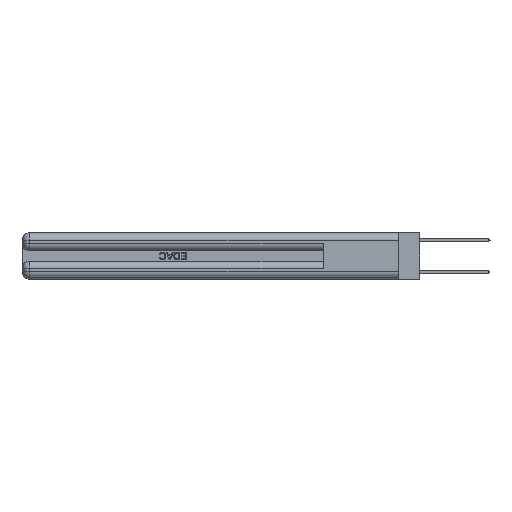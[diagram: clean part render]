
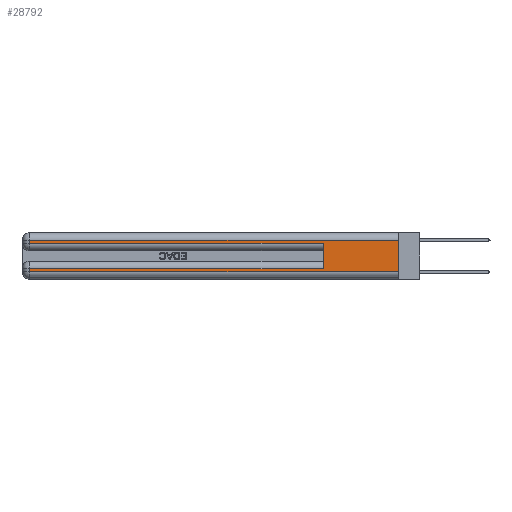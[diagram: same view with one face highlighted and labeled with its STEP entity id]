
A CAD part, left-side view. The second image highlights one B-rep face of the part: STEP entity #28792.
In plain terms, the highlighted planar face has unit normal (-1, 0, 0).
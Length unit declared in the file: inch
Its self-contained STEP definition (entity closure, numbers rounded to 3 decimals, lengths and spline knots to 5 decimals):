
#132 = LINE ( 'NONE', #19905, #26265 ) ;
#1682 = VERTEX_POINT ( 'NONE', #32365 ) ;
#1785 = ORIENTED_EDGE ( 'NONE', *, *, #12362, .T. ) ;
#2155 = EDGE_CURVE ( 'NONE', #25075, #1682, #28008, .T. ) ;
#2584 = LINE ( 'NONE', #23247, #15308 ) ;
#3776 = ORIENTED_EDGE ( 'NONE', *, *, #16377, .T. ) ;
#3825 = EDGE_CURVE ( 'NONE', #22819, #23001, #2584, .T. ) ;
#4511 = VERTEX_POINT ( 'NONE', #26385 ) ;
#4681 = DIRECTION ( 'NONE',  ( 0., 1., 0. ) ) ;
#5069 = EDGE_LOOP ( 'NONE', ( #28357, #23232, #3776, #12104, #25578, #13677, #1785, #31104 ) ) ;
#6188 = VERTEX_POINT ( 'NONE', #31157 ) ;
#6402 = CARTESIAN_POINT ( 'NONE',  ( 0., 0.6, 0.085 ) ) ;
#7669 = CARTESIAN_POINT ( 'NONE',  ( 0., 2.94, 0.06 ) ) ;
#7824 = VECTOR ( 'NONE', #28926, 39.37008 ) ;
#8677 = DIRECTION ( 'NONE',  ( 1., 0., 0. ) ) ;
#9078 = CARTESIAN_POINT ( 'NONE',  ( 0., 0., 0.06 ) ) ;
#10394 = LINE ( 'NONE', #29727, #29802 ) ;
#10498 = DIRECTION ( 'NONE',  ( 0., 0., 1. ) ) ;
#10641 = EDGE_CURVE ( 'NONE', #22819, #6188, #132, .T. ) ;
#10685 = LINE ( 'NONE', #29295, #30100 ) ;
#12054 = CARTESIAN_POINT ( 'NONE',  ( 0., 0.6, 0.285 ) ) ;
#12104 = ORIENTED_EDGE ( 'NONE', *, *, #23173, .T. ) ;
#12362 = EDGE_CURVE ( 'NONE', #6188, #28641, #14928, .T. ) ;
#13038 = AXIS2_PLACEMENT_3D ( 'NONE', #18746, #8677, #26354 ) ;
#13677 = ORIENTED_EDGE ( 'NONE', *, *, #10641, .T. ) ;
#14040 = EDGE_CURVE ( 'NONE', #28641, #18282, #28649, .T. ) ;
#14707 = EDGE_CURVE ( 'NONE', #25075, #18282, #10394, .T. ) ;
#14928 = LINE ( 'NONE', #30890, #26773 ) ;
#15273 = CARTESIAN_POINT ( 'NONE',  ( 0., 0., 0.285 ) ) ;
#15308 = VECTOR ( 'NONE', #10498, 39.37008 ) ;
#16315 = CARTESIAN_POINT ( 'NONE',  ( 0., 0., 0.31 ) ) ;
#16377 = EDGE_CURVE ( 'NONE', #1682, #4511, #10685, .T. ) ;
#17431 = CARTESIAN_POINT ( 'NONE',  ( 0., 0., 0.06 ) ) ;
#18282 = VERTEX_POINT ( 'NONE', #9078 ) ;
#18443 = LINE ( 'NONE', #15273, #24378 ) ;
#18746 = CARTESIAN_POINT ( 'NONE',  ( 0., 0., 0.37 ) ) ;
#19905 = CARTESIAN_POINT ( 'NONE',  ( 0., 0., 0.085 ) ) ;
#21131 = VECTOR ( 'NONE', #27491, 39.37008 ) ;
#22819 = VERTEX_POINT ( 'NONE', #6402 ) ;
#23001 = VERTEX_POINT ( 'NONE', #12054 ) ;
#23173 = EDGE_CURVE ( 'NONE', #4511, #23001, #18443, .T. ) ;
#23232 = ORIENTED_EDGE ( 'NONE', *, *, #2155, .T. ) ;
#23247 = CARTESIAN_POINT ( 'NONE',  ( 0., 0.6, 0.145 ) ) ;
#23386 = DIRECTION ( 'NONE',  ( 0., 0., -1. ) ) ;
#23843 = PLANE ( 'NONE',  #13038 ) ;
#24378 = VECTOR ( 'NONE', #27867, 39.37008 ) ;
#24775 = CARTESIAN_POINT ( 'NONE',  ( 0., 0., 0.31 ) ) ;
#25075 = VERTEX_POINT ( 'NONE', #24775 ) ;
#25578 = ORIENTED_EDGE ( 'NONE', *, *, #3825, .F. ) ;
#26265 = VECTOR ( 'NONE', #4681, 39.37008 ) ;
#26354 = DIRECTION ( 'NONE',  ( 0., 0., -1. ) ) ;
#26385 = CARTESIAN_POINT ( 'NONE',  ( 0., 2.94, 0.285 ) ) ;
#26773 = VECTOR ( 'NONE', #23386, 39.37008 ) ;
#27416 = FACE_OUTER_BOUND ( 'NONE', #5069, .T. ) ;
#27491 = DIRECTION ( 'NONE',  ( 0., -1., 0. ) ) ;
#27867 = DIRECTION ( 'NONE',  ( 0., -1., 0. ) ) ;
#28008 = LINE ( 'NONE', #16315, #7824 ) ;
#28357 = ORIENTED_EDGE ( 'NONE', *, *, #14707, .F. ) ;
#28641 = VERTEX_POINT ( 'NONE', #7669 ) ;
#28649 = LINE ( 'NONE', #17431, #21131 ) ;
#28792 = ADVANCED_FACE ( 'NONE', ( #27416 ), #23843, .F. ) ;
#28926 = DIRECTION ( 'NONE',  ( 0., 1., 0. ) ) ;
#29295 = CARTESIAN_POINT ( 'NONE',  ( 0., 2.94, 0.37 ) ) ;
#29727 = CARTESIAN_POINT ( 'NONE',  ( 0., 0., 0.37 ) ) ;
#29802 = VECTOR ( 'NONE', #32245, 39.37008 ) ;
#30100 = VECTOR ( 'NONE', #31813, 39.37008 ) ;
#30890 = CARTESIAN_POINT ( 'NONE',  ( 0., 2.94, 0.37 ) ) ;
#31104 = ORIENTED_EDGE ( 'NONE', *, *, #14040, .T. ) ;
#31157 = CARTESIAN_POINT ( 'NONE',  ( 0., 2.94, 0.085 ) ) ;
#31813 = DIRECTION ( 'NONE',  ( 0., 0., -1. ) ) ;
#32245 = DIRECTION ( 'NONE',  ( 0., 0., -1. ) ) ;
#32365 = CARTESIAN_POINT ( 'NONE',  ( 0., 2.94, 0.31 ) ) ;
